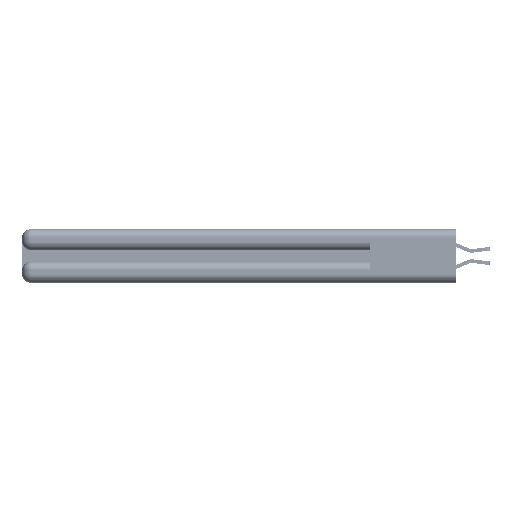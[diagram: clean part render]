
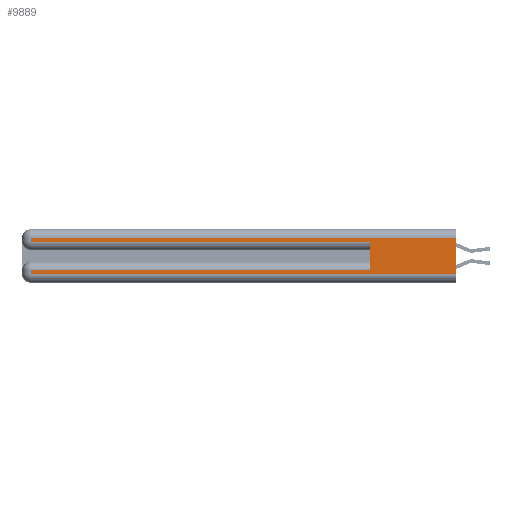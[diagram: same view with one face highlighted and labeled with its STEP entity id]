
A CAD part, left-side view. The second image highlights one B-rep face of the part: STEP entity #9889.
In plain terms, the highlighted planar face has unit normal (-1, 0, 0).
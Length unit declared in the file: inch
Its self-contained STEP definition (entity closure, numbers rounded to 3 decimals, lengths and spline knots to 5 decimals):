
#544 = VERTEX_POINT ( 'NONE', #27384 ) ;
#615 = ORIENTED_EDGE ( 'NONE', *, *, #37146, .T. ) ;
#1003 = ORIENTED_EDGE ( 'NONE', *, *, #13149, .T. ) ;
#2259 = AXIS2_PLACEMENT_3D ( 'NONE', #35501, #29522, #15813 ) ;
#3098 = VECTOR ( 'NONE', #13778, 39.37008 ) ;
#3340 = LINE ( 'NONE', #22369, #18960 ) ;
#5221 = VERTEX_POINT ( 'NONE', #28687 ) ;
#5580 = DIRECTION ( 'NONE',  ( 0., 0., -1. ) ) ;
#5769 = FACE_OUTER_BOUND ( 'NONE', #12725, .T. ) ;
#6092 = VECTOR ( 'NONE', #11806, 39.37008 ) ;
#7475 = EDGE_CURVE ( 'NONE', #36257, #8911, #24937, .T. ) ;
#8911 = VERTEX_POINT ( 'NONE', #10140 ) ;
#9692 = EDGE_CURVE ( 'NONE', #19431, #5221, #9694, .T. ) ;
#9694 = LINE ( 'NONE', #34656, #20114 ) ;
#9827 = VERTEX_POINT ( 'NONE', #20980 ) ;
#9889 = ADVANCED_FACE ( 'NONE', ( #5769 ), #25569, .F. ) ;
#10140 = CARTESIAN_POINT ( 'NONE',  ( 0., 2.94, 0.06 ) ) ;
#10671 = CARTESIAN_POINT ( 'NONE',  ( 0., 0.6, 0.145 ) ) ;
#11352 = DIRECTION ( 'NONE',  ( 0., 1., 0. ) ) ;
#11806 = DIRECTION ( 'NONE',  ( 0., 0., -1. ) ) ;
#12725 = EDGE_LOOP ( 'NONE', ( #25402, #615, #25459, #37430, #18082, #1003, #39976, #27774 ) ) ;
#13149 = EDGE_CURVE ( 'NONE', #9827, #36257, #3340, .T. ) ;
#13778 = DIRECTION ( 'NONE',  ( 0., 1., 0. ) ) ;
#14014 = CARTESIAN_POINT ( 'NONE',  ( 0., 0., 0.06 ) ) ;
#15446 = CARTESIAN_POINT ( 'NONE',  ( 0., 2.94, 0.37 ) ) ;
#15813 = DIRECTION ( 'NONE',  ( 0., 0., -1. ) ) ;
#16184 = VECTOR ( 'NONE', #30876, 39.37008 ) ;
#17091 = VECTOR ( 'NONE', #25201, 39.37008 ) ;
#17141 = LINE ( 'NONE', #33639, #3098 ) ;
#17170 = CARTESIAN_POINT ( 'NONE',  ( 0., 0., 0.06 ) ) ;
#17784 = DIRECTION ( 'NONE',  ( 0., -1., 0. ) ) ;
#18082 = ORIENTED_EDGE ( 'NONE', *, *, #22882, .F. ) ;
#18960 = VECTOR ( 'NONE', #11352, 39.37008 ) ;
#19431 = VERTEX_POINT ( 'NONE', #28360 ) ;
#20114 = VECTOR ( 'NONE', #31516, 39.37008 ) ;
#20980 = CARTESIAN_POINT ( 'NONE',  ( 0., 0.6, 0.085 ) ) ;
#21407 = LINE ( 'NONE', #10671, #16184 ) ;
#22369 = CARTESIAN_POINT ( 'NONE',  ( 0., 0., 0.085 ) ) ;
#22848 = EDGE_CURVE ( 'NONE', #8911, #36346, #33019, .T. ) ;
#22882 = EDGE_CURVE ( 'NONE', #9827, #5221, #21407, .T. ) ;
#23043 = EDGE_CURVE ( 'NONE', #544, #19431, #36216, .T. ) ;
#24613 = CARTESIAN_POINT ( 'NONE',  ( 0., 2.94, 0.085 ) ) ;
#24937 = LINE ( 'NONE', #15446, #17091 ) ;
#25201 = DIRECTION ( 'NONE',  ( 0., 0., -1. ) ) ;
#25402 = ORIENTED_EDGE ( 'NONE', *, *, #38679, .F. ) ;
#25459 = ORIENTED_EDGE ( 'NONE', *, *, #23043, .T. ) ;
#25569 = PLANE ( 'NONE',  #2259 ) ;
#26918 = LINE ( 'NONE', #41649, #6092 ) ;
#26952 = VECTOR ( 'NONE', #5580, 39.37008 ) ;
#27384 = CARTESIAN_POINT ( 'NONE',  ( 0., 2.94, 0.31 ) ) ;
#27774 = ORIENTED_EDGE ( 'NONE', *, *, #22848, .T. ) ;
#28360 = CARTESIAN_POINT ( 'NONE',  ( 0., 2.94, 0.285 ) ) ;
#28687 = CARTESIAN_POINT ( 'NONE',  ( 0., 0.6, 0.285 ) ) ;
#29522 = DIRECTION ( 'NONE',  ( 1., 0., 0. ) ) ;
#30876 = DIRECTION ( 'NONE',  ( 0., 0., 1. ) ) ;
#31516 = DIRECTION ( 'NONE',  ( 0., -1., 0. ) ) ;
#31564 = VERTEX_POINT ( 'NONE', #34813 ) ;
#33019 = LINE ( 'NONE', #14014, #41205 ) ;
#33639 = CARTESIAN_POINT ( 'NONE',  ( 0., 0., 0.31 ) ) ;
#34656 = CARTESIAN_POINT ( 'NONE',  ( 0., 0., 0.285 ) ) ;
#34813 = CARTESIAN_POINT ( 'NONE',  ( 0., 0., 0.31 ) ) ;
#35501 = CARTESIAN_POINT ( 'NONE',  ( 0., 0., 0.37 ) ) ;
#36216 = LINE ( 'NONE', #38609, #26952 ) ;
#36257 = VERTEX_POINT ( 'NONE', #24613 ) ;
#36346 = VERTEX_POINT ( 'NONE', #17170 ) ;
#37146 = EDGE_CURVE ( 'NONE', #31564, #544, #17141, .T. ) ;
#37430 = ORIENTED_EDGE ( 'NONE', *, *, #9692, .T. ) ;
#38609 = CARTESIAN_POINT ( 'NONE',  ( 0., 2.94, 0.37 ) ) ;
#38679 = EDGE_CURVE ( 'NONE', #31564, #36346, #26918, .T. ) ;
#39976 = ORIENTED_EDGE ( 'NONE', *, *, #7475, .T. ) ;
#41205 = VECTOR ( 'NONE', #17784, 39.37008 ) ;
#41649 = CARTESIAN_POINT ( 'NONE',  ( 0., 0., 0.37 ) ) ;
